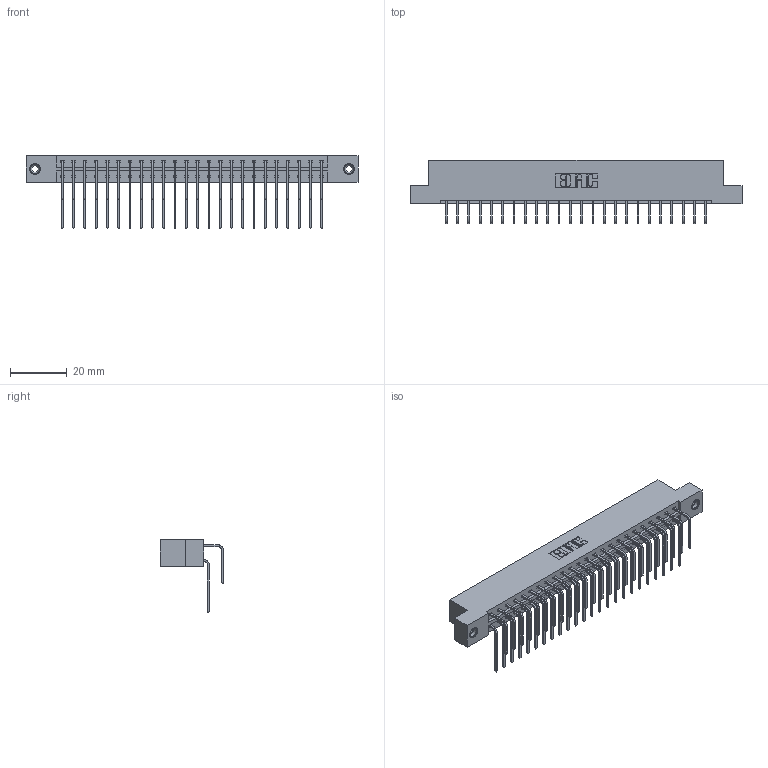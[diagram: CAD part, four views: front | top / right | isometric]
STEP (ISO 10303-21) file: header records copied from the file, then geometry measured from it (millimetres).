
FILE_DESCRIPTION (( 'STEP AP203' ), '1' );
FILE_NAME ('333-048-558-208.STEP', '2018-08-04T00:06:07', ( '' ), ( '' ), 'SwSTEP 2.0', 'SolidWorks 2016', '' );
FILE_SCHEMA (( 'CONFIG_CONTROL_DESIGN' ));
Length unit declared in the file: inch
Products named in the file (5): 333-048-558-208; 333 Part_Flush - .156 Dia - TI; 345-292-001_558 559 Tail - 1; 345-292-001_558 Tail - 2; 345-250-001_345-250-003-102
Assembly tree (51 placements, depth 2):
  333-048-558-208
    333 Part_Flush - .156 Dia - TI
    345-292-001_558 559 Tail - 1  x24
    345-292-001_558 Tail - 2  x24
    345-250-001_345-250-003-102  x2
Bounding box: 116.64 x 22.17 x 25.53 mm (x, y, z)
Volume: 12010 mm3; surface area: 15406.4 mm2
Topology: 51 solids, 51 shells, 2766 faces, 8175 edges, 5378 vertices
Faces by surface type: plane 1926, cylinder 824, cone 12, torus 4
Entity records: 20738 total; most frequent: CARTESIAN_POINT 3492, ORIENTED_EDGE 3370, DIRECTION 3027, EDGE_CURVE 1685, VECTOR 1497, LINE 1497, VERTEX_POINT 1116, AXIS2_PLACEMENT_3D 765
